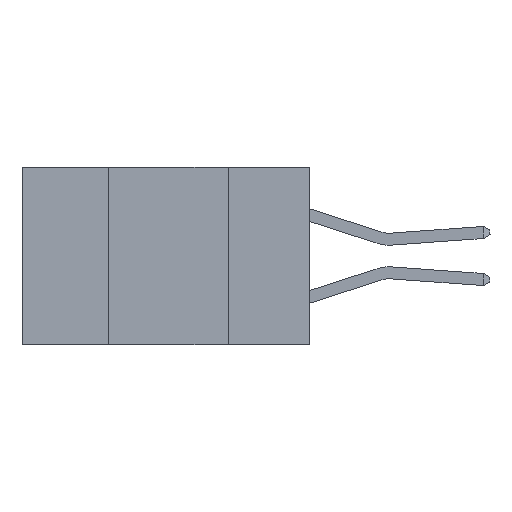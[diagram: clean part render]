
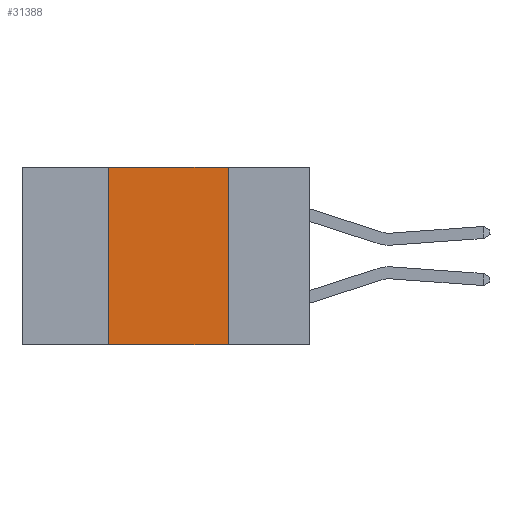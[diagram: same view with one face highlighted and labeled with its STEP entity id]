
A CAD part, left-side view. The second image highlights one B-rep face of the part: STEP entity #31388.
In plain terms, the highlighted planar face has unit normal (-1, 0, 0).
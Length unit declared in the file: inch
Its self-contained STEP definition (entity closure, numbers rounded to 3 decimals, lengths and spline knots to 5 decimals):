
#2121 = CARTESIAN_POINT ( 'NONE',  ( 0., 0.42, -0.37 ) ) ;
#3998 = CARTESIAN_POINT ( 'NONE',  ( 0., 0.17, 0. ) ) ;
#4181 = CARTESIAN_POINT ( 'NONE',  ( 0., 0.42, 0. ) ) ;
#5751 = EDGE_CURVE ( 'NONE', #21806, #20428, #8812, .T. ) ;
#6545 = LINE ( 'NONE', #32876, #19951 ) ;
#7689 = LINE ( 'NONE', #31543, #13995 ) ;
#7774 = CARTESIAN_POINT ( 'NONE',  ( 0., 0.17, -0.37 ) ) ;
#7853 = EDGE_CURVE ( 'NONE', #14551, #24379, #6545, .T. ) ;
#8812 = LINE ( 'NONE', #23522, #22979 ) ;
#9364 = CARTESIAN_POINT ( 'NONE',  ( 0., 0.6, 0. ) ) ;
#9440 = DIRECTION ( 'NONE',  ( 0., 0., -1. ) ) ;
#11577 = AXIS2_PLACEMENT_3D ( 'NONE', #9364, #28017, #12044 ) ;
#12044 = DIRECTION ( 'NONE',  ( 0., 0., -1. ) ) ;
#13117 = EDGE_CURVE ( 'NONE', #14551, #21806, #7689, .T. ) ;
#13995 = VECTOR ( 'NONE', #23572, 39.37008 ) ;
#14375 = EDGE_CURVE ( 'NONE', #20428, #24379, #19197, .T. ) ;
#14551 = VERTEX_POINT ( 'NONE', #2121 ) ;
#15079 = CARTESIAN_POINT ( 'NONE',  ( 0., 0.17, 0. ) ) ;
#16885 = DIRECTION ( 'NONE',  ( 0., -1., 0. ) ) ;
#19197 = LINE ( 'NONE', #3998, #26275 ) ;
#19951 = VECTOR ( 'NONE', #16885, 39.37008 ) ;
#19974 = PLANE ( 'NONE',  #11577 ) ;
#20428 = VERTEX_POINT ( 'NONE', #15079 ) ;
#21806 = VERTEX_POINT ( 'NONE', #4181 ) ;
#22979 = VECTOR ( 'NONE', #34155, 39.37008 ) ;
#23447 = ORIENTED_EDGE ( 'NONE', *, *, #14375, .F. ) ;
#23522 = CARTESIAN_POINT ( 'NONE',  ( 0., 0.6, 0. ) ) ;
#23572 = DIRECTION ( 'NONE',  ( 0., 0., 1. ) ) ;
#24254 = ORIENTED_EDGE ( 'NONE', *, *, #5751, .F. ) ;
#24379 = VERTEX_POINT ( 'NONE', #7774 ) ;
#24449 = ORIENTED_EDGE ( 'NONE', *, *, #13117, .F. ) ;
#25343 = ORIENTED_EDGE ( 'NONE', *, *, #7853, .T. ) ;
#26275 = VECTOR ( 'NONE', #9440, 39.37008 ) ;
#28017 = DIRECTION ( 'NONE',  ( 1., 0., 0. ) ) ;
#28856 = FACE_OUTER_BOUND ( 'NONE', #33984, .T. ) ;
#31388 = ADVANCED_FACE ( 'NONE', ( #28856 ), #19974, .F. ) ;
#31543 = CARTESIAN_POINT ( 'NONE',  ( 0., 0.42, 0. ) ) ;
#32876 = CARTESIAN_POINT ( 'NONE',  ( 0., 0.6, -0.37 ) ) ;
#33984 = EDGE_LOOP ( 'NONE', ( #23447, #24254, #24449, #25343 ) ) ;
#34155 = DIRECTION ( 'NONE',  ( 0., -1., 0. ) ) ;
